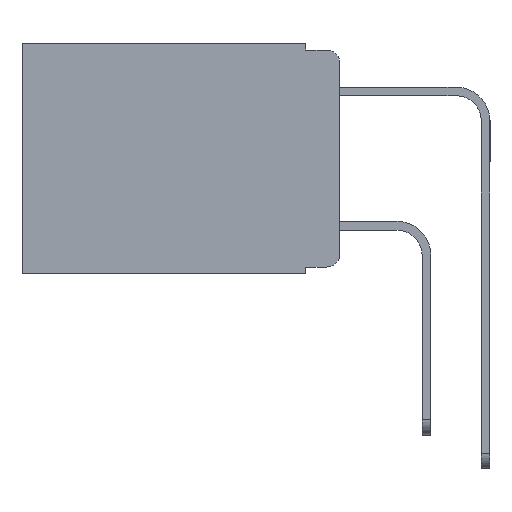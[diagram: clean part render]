
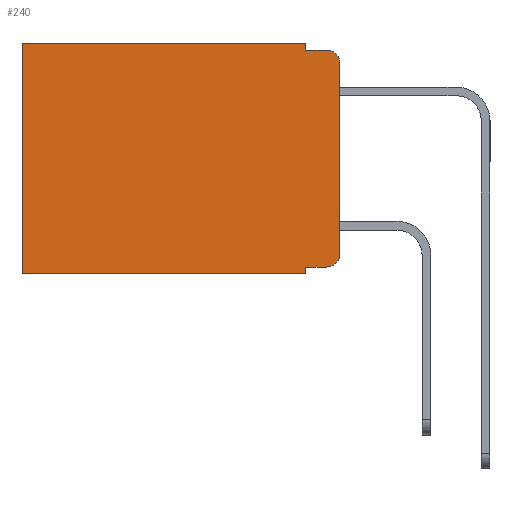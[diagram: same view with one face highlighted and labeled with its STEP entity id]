
A CAD part, left-side view. The second image highlights one B-rep face of the part: STEP entity #240.
In plain terms, the highlighted planar face has unit normal (-1, 0, 0).
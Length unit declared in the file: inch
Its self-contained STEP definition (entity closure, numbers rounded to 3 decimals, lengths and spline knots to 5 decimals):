
#216 = CARTESIAN_POINT ( 'NONE',  ( 0.298, 0.02, -0.313 ) ) ;
#240 = ADVANCED_FACE ( 'NONE', ( #2141 ), #7324, .F. ) ;
#270 = DIRECTION ( 'NONE',  ( -1., 0., 0. ) ) ;
#281 = CARTESIAN_POINT ( 'NONE',  ( 0.298, 0., -0.313 ) ) ;
#339 = ORIENTED_EDGE ( 'NONE', *, *, #10102, .T. ) ;
#502 = LINE ( 'NONE', #9179, #6978 ) ;
#928 = CARTESIAN_POINT ( 'NONE',  ( 0.298, 0.051, -0.01 ) ) ;
#1133 = VERTEX_POINT ( 'NONE', #12501 ) ;
#1418 = CARTESIAN_POINT ( 'NONE',  ( 0.298, 0., -0.03 ) ) ;
#1611 = CARTESIAN_POINT ( 'NONE',  ( 0.298, 0.051, -0.333 ) ) ;
#1785 = VERTEX_POINT ( 'NONE', #5035 ) ;
#1792 = CARTESIAN_POINT ( 'NONE',  ( 0.298, 0.051, 0. ) ) ;
#1978 = CARTESIAN_POINT ( 'NONE',  ( 0.298, 0.051, -0.01 ) ) ;
#1992 = ORIENTED_EDGE ( 'NONE', *, *, #8434, .T. ) ;
#2058 = AXIS2_PLACEMENT_3D ( 'NONE', #216, #270, #3702 ) ;
#2141 = FACE_OUTER_BOUND ( 'NONE', #12335, .T. ) ;
#2272 = CARTESIAN_POINT ( 'NONE',  ( 0.298, 0.473, 0. ) ) ;
#2347 = DIRECTION ( 'NONE',  ( 0., 0., -1. ) ) ;
#2363 = VERTEX_POINT ( 'NONE', #13484 ) ;
#2468 = DIRECTION ( 'NONE',  ( 0., 0., -1. ) ) ;
#2866 = ORIENTED_EDGE ( 'NONE', *, *, #9777, .F. ) ;
#3129 = EDGE_CURVE ( 'NONE', #7875, #8561, #9540, .T. ) ;
#3548 = DIRECTION ( 'NONE',  ( -1., 0., 0. ) ) ;
#3702 = DIRECTION ( 'NONE',  ( 0., 0., -1. ) ) ;
#3854 = EDGE_CURVE ( 'NONE', #5242, #7875, #9628, .T. ) ;
#4620 = CARTESIAN_POINT ( 'NONE',  ( 0.298, 0.051, 0. ) ) ;
#4656 = EDGE_CURVE ( 'NONE', #5242, #1785, #502, .T. ) ;
#4888 = ORIENTED_EDGE ( 'NONE', *, *, #5406, .T. ) ;
#4939 = VECTOR ( 'NONE', #13547, 39.37008 ) ;
#4964 = CARTESIAN_POINT ( 'NONE',  ( 0.298, 0.473, 0. ) ) ;
#5031 = LINE ( 'NONE', #9038, #12833 ) ;
#5035 = CARTESIAN_POINT ( 'NONE',  ( 0.298, 0.051, -0.343 ) ) ;
#5242 = VERTEX_POINT ( 'NONE', #1611 ) ;
#5406 = EDGE_CURVE ( 'NONE', #11001, #2363, #9931, .T. ) ;
#5416 = VERTEX_POINT ( 'NONE', #1418 ) ;
#6179 = ORIENTED_EDGE ( 'NONE', *, *, #4656, .F. ) ;
#6193 = EDGE_CURVE ( 'NONE', #8389, #6752, #8156, .T. ) ;
#6239 = VECTOR ( 'NONE', #12840, 39.37008 ) ;
#6271 = ORIENTED_EDGE ( 'NONE', *, *, #6193, .F. ) ;
#6581 = LINE ( 'NONE', #11917, #6239 ) ;
#6752 = VERTEX_POINT ( 'NONE', #1978 ) ;
#6961 = EDGE_CURVE ( 'NONE', #6752, #1133, #10307, .T. ) ;
#6978 = VECTOR ( 'NONE', #13522, 39.37008 ) ;
#7043 = DIRECTION ( 'NONE',  ( 0., 0., -1. ) ) ;
#7165 = VECTOR ( 'NONE', #8531, 39.37008 ) ;
#7324 = PLANE ( 'NONE',  #11177 ) ;
#7837 = VECTOR ( 'NONE', #7043, 39.37008 ) ;
#7875 = VERTEX_POINT ( 'NONE', #10120 ) ;
#8136 = ORIENTED_EDGE ( 'NONE', *, *, #3854, .T. ) ;
#8156 = LINE ( 'NONE', #1792, #7837 ) ;
#8389 = VERTEX_POINT ( 'NONE', #4620 ) ;
#8434 = EDGE_CURVE ( 'NONE', #5416, #1133, #12582, .T. ) ;
#8531 = DIRECTION ( 'NONE',  ( 0., 0., -1. ) ) ;
#8561 = VERTEX_POINT ( 'NONE', #281 ) ;
#8783 = DIRECTION ( 'NONE',  ( 1., 0., 0. ) ) ;
#9038 = CARTESIAN_POINT ( 'NONE',  ( 0.298, 0., 0. ) ) ;
#9179 = CARTESIAN_POINT ( 'NONE',  ( 0.298, 0.051, 0. ) ) ;
#9389 = ORIENTED_EDGE ( 'NONE', *, *, #13251, .F. ) ;
#9423 = CARTESIAN_POINT ( 'NONE',  ( 0.298, 0., 0. ) ) ;
#9540 = CIRCLE ( 'NONE', #2058, 0.02 ) ;
#9628 = LINE ( 'NONE', #11128, #11536 ) ;
#9683 = VECTOR ( 'NONE', #10394, 39.37008 ) ;
#9777 = EDGE_CURVE ( 'NONE', #5416, #8561, #5031, .T. ) ;
#9931 = LINE ( 'NONE', #2272, #7165 ) ;
#10102 = EDGE_CURVE ( 'NONE', #8389, #11001, #12154, .T. ) ;
#10103 = CARTESIAN_POINT ( 'NONE',  ( 0.298, 0.02, -0.03 ) ) ;
#10120 = CARTESIAN_POINT ( 'NONE',  ( 0.298, 0.02, -0.333 ) ) ;
#10307 = LINE ( 'NONE', #928, #4939 ) ;
#10394 = DIRECTION ( 'NONE',  ( 0., 1., 0. ) ) ;
#11001 = VERTEX_POINT ( 'NONE', #4964 ) ;
#11051 = DIRECTION ( 'NONE',  ( 0., 0., -1. ) ) ;
#11128 = CARTESIAN_POINT ( 'NONE',  ( 0.298, 0.051, -0.333 ) ) ;
#11149 = ORIENTED_EDGE ( 'NONE', *, *, #6961, .F. ) ;
#11177 = AXIS2_PLACEMENT_3D ( 'NONE', #12528, #8783, #2468 ) ;
#11536 = VECTOR ( 'NONE', #12911, 39.37008 ) ;
#11917 = CARTESIAN_POINT ( 'NONE',  ( 0.298, 0., -0.343 ) ) ;
#12154 = LINE ( 'NONE', #9423, #9683 ) ;
#12335 = EDGE_LOOP ( 'NONE', ( #2866, #1992, #11149, #6271, #339, #4888, #9389, #6179, #8136, #12806 ) ) ;
#12501 = CARTESIAN_POINT ( 'NONE',  ( 0.298, 0.02, -0.01 ) ) ;
#12528 = CARTESIAN_POINT ( 'NONE',  ( 0.298, 0., 0. ) ) ;
#12582 = CIRCLE ( 'NONE', #13614, 0.02 ) ;
#12806 = ORIENTED_EDGE ( 'NONE', *, *, #3129, .T. ) ;
#12833 = VECTOR ( 'NONE', #2347, 39.37008 ) ;
#12840 = DIRECTION ( 'NONE',  ( 0., 1., 0. ) ) ;
#12911 = DIRECTION ( 'NONE',  ( 0., -1., 0. ) ) ;
#13251 = EDGE_CURVE ( 'NONE', #1785, #2363, #6581, .T. ) ;
#13484 = CARTESIAN_POINT ( 'NONE',  ( 0.298, 0.473, -0.343 ) ) ;
#13522 = DIRECTION ( 'NONE',  ( 0., 0., -1. ) ) ;
#13547 = DIRECTION ( 'NONE',  ( 0., -1., 0. ) ) ;
#13614 = AXIS2_PLACEMENT_3D ( 'NONE', #10103, #3548, #11051 ) ;
